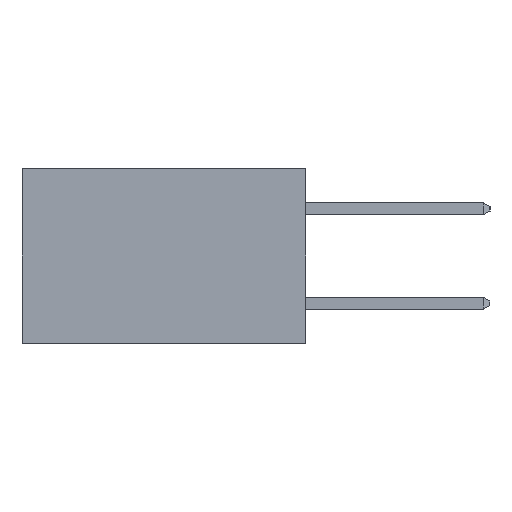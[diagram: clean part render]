
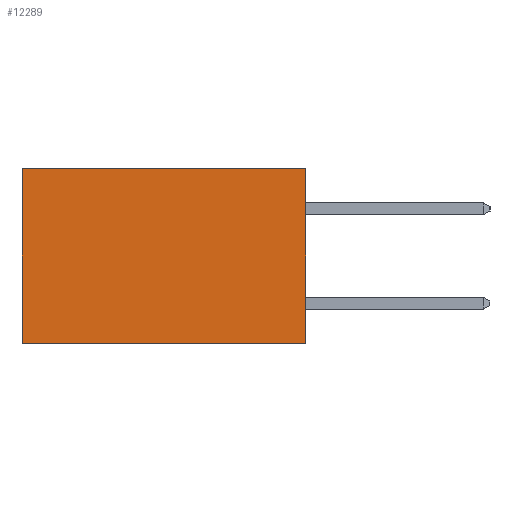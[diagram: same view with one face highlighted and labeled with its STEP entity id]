
A CAD part, left-side view. The second image highlights one B-rep face of the part: STEP entity #12289.
In plain terms, the highlighted planar face has unit normal (-1, 0, 0).
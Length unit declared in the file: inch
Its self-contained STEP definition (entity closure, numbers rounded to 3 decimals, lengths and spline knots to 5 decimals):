
#432 = VECTOR ( 'NONE', #14082, 39.37008 ) ;
#1541 = AXIS2_PLACEMENT_3D ( 'NONE', #7230, #16853, #7303 ) ;
#1728 = EDGE_CURVE ( 'NONE', #6800, #6287, #19180, .T. ) ;
#2126 = CARTESIAN_POINT ( 'NONE',  ( 0.298, 0., 0. ) ) ;
#2626 = VECTOR ( 'NONE', #20549, 39.37008 ) ;
#3110 = CARTESIAN_POINT ( 'NONE',  ( 0.298, 0.6, 0. ) ) ;
#3119 = VECTOR ( 'NONE', #10371, 39.37008 ) ;
#3132 = EDGE_CURVE ( 'NONE', #6565, #6800, #10174, .T. ) ;
#4991 = EDGE_LOOP ( 'NONE', ( #7702, #5808, #8180, #13556 ) ) ;
#5633 = CARTESIAN_POINT ( 'NONE',  ( 0.298, 0., -0.37 ) ) ;
#5651 = PLANE ( 'NONE',  #1541 ) ;
#5808 = ORIENTED_EDGE ( 'NONE', *, *, #15910, .F. ) ;
#6287 = VERTEX_POINT ( 'NONE', #6313 ) ;
#6313 = CARTESIAN_POINT ( 'NONE',  ( 0.298, 0.6, -0.37 ) ) ;
#6565 = VERTEX_POINT ( 'NONE', #2126 ) ;
#6800 = VERTEX_POINT ( 'NONE', #3110 ) ;
#7230 = CARTESIAN_POINT ( 'NONE',  ( 0.298, 0., 0. ) ) ;
#7303 = DIRECTION ( 'NONE',  ( 0., 0., -1. ) ) ;
#7465 = CARTESIAN_POINT ( 'NONE',  ( 0.298, 0.6, 0. ) ) ;
#7702 = ORIENTED_EDGE ( 'NONE', *, *, #1728, .T. ) ;
#8180 = ORIENTED_EDGE ( 'NONE', *, *, #13857, .F. ) ;
#9178 = VECTOR ( 'NONE', #9812, 39.37008 ) ;
#9812 = DIRECTION ( 'NONE',  ( 0., 1., 0. ) ) ;
#10174 = LINE ( 'NONE', #18502, #9178 ) ;
#10371 = DIRECTION ( 'NONE',  ( 0., 1., 0. ) ) ;
#12289 = ADVANCED_FACE ( 'NONE', ( #17852 ), #5651, .F. ) ;
#12547 = CARTESIAN_POINT ( 'NONE',  ( 0.298, 0., 0. ) ) ;
#13556 = ORIENTED_EDGE ( 'NONE', *, *, #3132, .T. ) ;
#13593 = CARTESIAN_POINT ( 'NONE',  ( 0.298, 0., -0.37 ) ) ;
#13857 = EDGE_CURVE ( 'NONE', #6565, #20037, #20673, .T. ) ;
#14082 = DIRECTION ( 'NONE',  ( 0., 0., -1. ) ) ;
#15910 = EDGE_CURVE ( 'NONE', #20037, #6287, #15991, .T. ) ;
#15991 = LINE ( 'NONE', #13593, #3119 ) ;
#16853 = DIRECTION ( 'NONE',  ( 1., 0., 0. ) ) ;
#17852 = FACE_OUTER_BOUND ( 'NONE', #4991, .T. ) ;
#18502 = CARTESIAN_POINT ( 'NONE',  ( 0.298, 0., 0. ) ) ;
#19180 = LINE ( 'NONE', #7465, #2626 ) ;
#20037 = VERTEX_POINT ( 'NONE', #5633 ) ;
#20549 = DIRECTION ( 'NONE',  ( 0., 0., -1. ) ) ;
#20673 = LINE ( 'NONE', #12547, #432 ) ;
